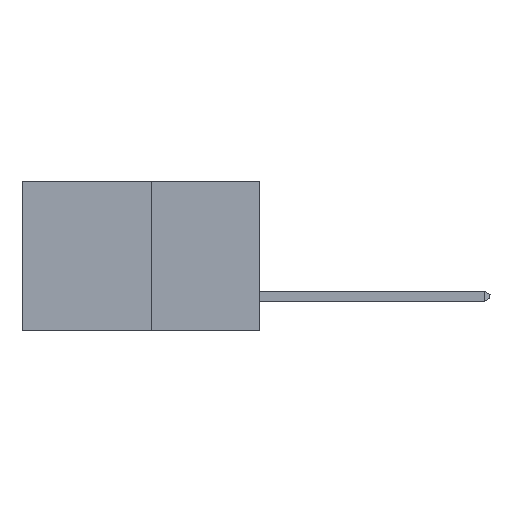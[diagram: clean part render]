
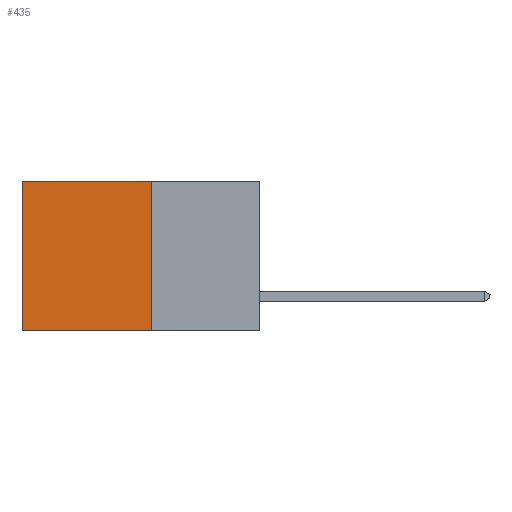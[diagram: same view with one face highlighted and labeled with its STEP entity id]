
A CAD part, left-side view. The second image highlights one B-rep face of the part: STEP entity #435.
In plain terms, the highlighted planar face has unit normal (-1, 0, 0).
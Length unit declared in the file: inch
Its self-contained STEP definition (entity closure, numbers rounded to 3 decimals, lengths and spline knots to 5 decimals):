
#195 = CARTESIAN_POINT ( 'NONE',  ( 0.277, 0.59, -0.37 ) ) ;
#435 = ADVANCED_FACE ( 'NONE', ( #8199 ), #9868, .F. ) ;
#565 = DIRECTION ( 'NONE',  ( 0., 0., -1. ) ) ;
#814 = VECTOR ( 'NONE', #11945, 39.37008 ) ;
#898 = DIRECTION ( 'NONE',  ( 0., 1., 0. ) ) ;
#1436 = EDGE_LOOP ( 'NONE', ( #11131, #4323, #9246, #2465 ) ) ;
#1965 = VERTEX_POINT ( 'NONE', #195 ) ;
#2188 = CARTESIAN_POINT ( 'NONE',  ( 0.277, 0.27, -0.37 ) ) ;
#2465 = ORIENTED_EDGE ( 'NONE', *, *, #12215, .T. ) ;
#3304 = CARTESIAN_POINT ( 'NONE',  ( 0.277, 0.27, -0.37 ) ) ;
#4323 = ORIENTED_EDGE ( 'NONE', *, *, #8691, .F. ) ;
#5468 = LINE ( 'NONE', #11435, #8313 ) ;
#5719 = AXIS2_PLACEMENT_3D ( 'NONE', #11235, #9982, #10776 ) ;
#7325 = VECTOR ( 'NONE', #898, 39.37008 ) ;
#7671 = LINE ( 'NONE', #13712, #7325 ) ;
#8199 = FACE_OUTER_BOUND ( 'NONE', #1436, .T. ) ;
#8313 = VECTOR ( 'NONE', #12487, 39.37008 ) ;
#8395 = EDGE_CURVE ( 'NONE', #11921, #12344, #11632, .T. ) ;
#8691 = EDGE_CURVE ( 'NONE', #12344, #1965, #5468, .T. ) ;
#9084 = CARTESIAN_POINT ( 'NONE',  ( 0.277, 0.27, 0. ) ) ;
#9246 = ORIENTED_EDGE ( 'NONE', *, *, #8395, .F. ) ;
#9868 = PLANE ( 'NONE',  #5719 ) ;
#9982 = DIRECTION ( 'NONE',  ( 1., 0., 0. ) ) ;
#10585 = LINE ( 'NONE', #13402, #13039 ) ;
#10619 = VERTEX_POINT ( 'NONE', #12754 ) ;
#10776 = DIRECTION ( 'NONE',  ( 0., 0., -1. ) ) ;
#11131 = ORIENTED_EDGE ( 'NONE', *, *, #12042, .T. ) ;
#11235 = CARTESIAN_POINT ( 'NONE',  ( 0.277, 0.27, -0.37 ) ) ;
#11435 = CARTESIAN_POINT ( 'NONE',  ( 0.277, 0.27, -0.37 ) ) ;
#11632 = LINE ( 'NONE', #2188, #814 ) ;
#11921 = VERTEX_POINT ( 'NONE', #9084 ) ;
#11945 = DIRECTION ( 'NONE',  ( 0., 0., -1. ) ) ;
#12042 = EDGE_CURVE ( 'NONE', #10619, #1965, #10585, .T. ) ;
#12215 = EDGE_CURVE ( 'NONE', #11921, #10619, #7671, .T. ) ;
#12344 = VERTEX_POINT ( 'NONE', #3304 ) ;
#12487 = DIRECTION ( 'NONE',  ( 0., 1., 0. ) ) ;
#12754 = CARTESIAN_POINT ( 'NONE',  ( 0.277, 0.59, 0. ) ) ;
#13039 = VECTOR ( 'NONE', #565, 39.37008 ) ;
#13402 = CARTESIAN_POINT ( 'NONE',  ( 0.277, 0.59, -0.37 ) ) ;
#13712 = CARTESIAN_POINT ( 'NONE',  ( 0.277, 0.27, 0. ) ) ;
